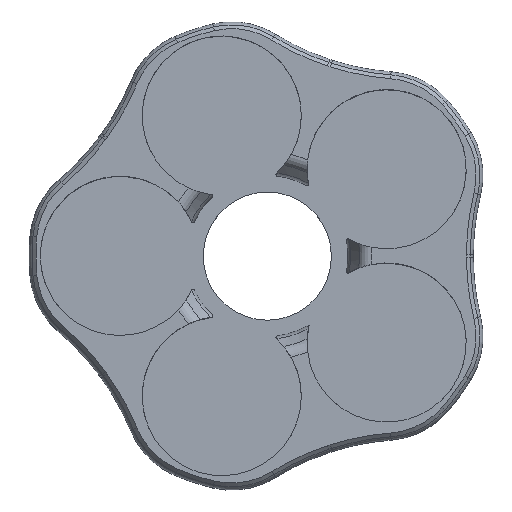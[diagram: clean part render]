
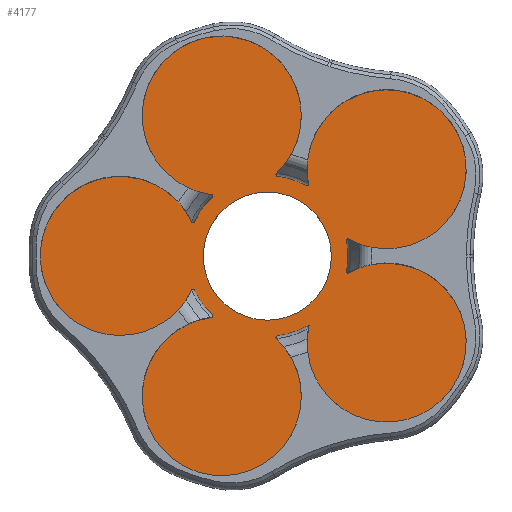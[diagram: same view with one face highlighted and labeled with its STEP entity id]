
A CAD part, top view. The second image highlights one B-rep face of the part: STEP entity #4177.
In plain terms, the highlighted planar face has unit normal (0, 0, 1).
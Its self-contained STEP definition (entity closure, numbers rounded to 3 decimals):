
#107=FACE_BOUND('',#1178,.T.);
#131=PLANE('',#4820);
#906=FACE_OUTER_BOUND('',#1177,.T.);
#1177=EDGE_LOOP('',(#3790,#3791,#3792,#3793,#3794,#3795,#3796,#3797,#3798,
#3799,#3800,#3801,#3802,#3803,#3804,#3805,#3806,#3807,#3808));
#1178=EDGE_LOOP('',(#3809));
#1285=CIRCLE('',#4345,0.1);
#1289=CIRCLE('',#4350,5.775);
#1294=CIRCLE('',#4357,0.1);
#1295=CIRCLE('',#4359,5.775);
#1299=CIRCLE('',#4364,0.1);
#1301=CIRCLE('',#4367,0.1);
#1303=CIRCLE('',#4370,5.85);
#1310=CIRCLE('',#4381,5.775);
#1318=CIRCLE('',#4398,5.775);
#1322=CIRCLE('',#4403,0.1);
#1326=CIRCLE('',#4409,0.1);
#1332=CIRCLE('',#4420,0.1);
#1334=CIRCLE('',#4423,5.85);
#1336=CIRCLE('',#4426,0.1);
#1341=CIRCLE('',#4433,0.1);
#1343=CIRCLE('',#4436,5.775);
#1549=CIRCLE('',#4793,4.65);
#1553=CIRCLE('',#4801,5.85);
#1556=CIRCLE('',#4808,5.85);
#1558=CIRCLE('',#4812,5.85);
#1645=VERTEX_POINT('',#6530);
#1646=VERTEX_POINT('',#6532);
#1662=VERTEX_POINT('',#6606);
#1666=VERTEX_POINT('',#6618);
#1667=VERTEX_POINT('',#6620);
#1668=VERTEX_POINT('',#6624);
#1684=VERTEX_POINT('',#6698);
#1687=VERTEX_POINT('',#6705);
#1688=VERTEX_POINT('',#6707);
#1710=VERTEX_POINT('',#6853);
#1729=VERTEX_POINT('',#7000);
#1730=VERTEX_POINT('',#7002);
#1742=VERTEX_POINT('',#7058);
#1744=VERTEX_POINT('',#7067);
#1756=VERTEX_POINT('',#7138);
#1757=VERTEX_POINT('',#7140);
#1759=VERTEX_POINT('',#7149);
#1763=VERTEX_POINT('',#7161);
#1764=VERTEX_POINT('',#7163);
#1931=VERTEX_POINT('',#8048);
#2060=EDGE_CURVE('',#1645,#1646,#1285,.F.);
#2078=EDGE_CURVE('',#1645,#1662,#1289,.T.);
#2084=EDGE_CURVE('',#1666,#1667,#1294,.F.);
#2086=EDGE_CURVE('',#1668,#1667,#1295,.T.);
#2104=EDGE_CURVE('',#1684,#1662,#1299,.F.);
#2107=EDGE_CURVE('',#1687,#1688,#1301,.F.);
#2110=EDGE_CURVE('',#1688,#1684,#1303,.T.);
#2138=EDGE_CURVE('',#1687,#1710,#1310,.T.);
#2167=EDGE_CURVE('',#1730,#1729,#1318,.T.);
#2181=EDGE_CURVE('',#1742,#1729,#1322,.F.);
#2186=EDGE_CURVE('',#1744,#1710,#1326,.F.);
#2202=EDGE_CURVE('',#1756,#1757,#1332,.F.);
#2205=EDGE_CURVE('',#1757,#1744,#1334,.T.);
#2207=EDGE_CURVE('',#1730,#1759,#1336,.F.);
#2214=EDGE_CURVE('',#1763,#1764,#1341,.F.);
#2225=EDGE_CURVE('',#1756,#1764,#1343,.T.);
#2549=EDGE_CURVE('',#1931,#1931,#1549,.T.);
#2553=EDGE_CURVE('',#1646,#1666,#1553,.T.);
#2556=EDGE_CURVE('',#1668,#1742,#1556,.T.);
#2558=EDGE_CURVE('',#1759,#1763,#1558,.T.);
#3790=ORIENTED_EDGE('',*,*,#2138,.T.);
#3791=ORIENTED_EDGE('',*,*,#2186,.F.);
#3792=ORIENTED_EDGE('',*,*,#2205,.F.);
#3793=ORIENTED_EDGE('',*,*,#2202,.F.);
#3794=ORIENTED_EDGE('',*,*,#2225,.T.);
#3795=ORIENTED_EDGE('',*,*,#2214,.F.);
#3796=ORIENTED_EDGE('',*,*,#2558,.F.);
#3797=ORIENTED_EDGE('',*,*,#2207,.F.);
#3798=ORIENTED_EDGE('',*,*,#2167,.T.);
#3799=ORIENTED_EDGE('',*,*,#2181,.F.);
#3800=ORIENTED_EDGE('',*,*,#2556,.F.);
#3801=ORIENTED_EDGE('',*,*,#2086,.T.);
#3802=ORIENTED_EDGE('',*,*,#2084,.F.);
#3803=ORIENTED_EDGE('',*,*,#2553,.F.);
#3804=ORIENTED_EDGE('',*,*,#2060,.F.);
#3805=ORIENTED_EDGE('',*,*,#2078,.T.);
#3806=ORIENTED_EDGE('',*,*,#2104,.F.);
#3807=ORIENTED_EDGE('',*,*,#2110,.F.);
#3808=ORIENTED_EDGE('',*,*,#2107,.F.);
#3809=ORIENTED_EDGE('',*,*,#2549,.F.);
#4177=ADVANCED_FACE('',(#906,#107),#131,.T.);
#4345=AXIS2_PLACEMENT_3D('',#6533,#5151,#5152);
#4350=AXIS2_PLACEMENT_3D('',#6608,#5167,#5168);
#4357=AXIS2_PLACEMENT_3D('',#6621,#5182,#5183);
#4359=AXIS2_PLACEMENT_3D('',#6625,#5187,#5188);
#4364=AXIS2_PLACEMENT_3D('',#6700,#5203,#5204);
#4367=AXIS2_PLACEMENT_3D('',#6708,#5210,#5211);
#4370=AXIS2_PLACEMENT_3D('',#6712,#5217,#5218);
#4381=AXIS2_PLACEMENT_3D('',#6855,#5246,#5247);
#4398=AXIS2_PLACEMENT_3D('',#7003,#5287,#5288);
#4403=AXIS2_PLACEMENT_3D('',#7060,#5301,#5302);
#4409=AXIS2_PLACEMENT_3D('',#7069,#5314,#5315);
#4420=AXIS2_PLACEMENT_3D('',#7141,#5340,#5341);
#4423=AXIS2_PLACEMENT_3D('',#7145,#5347,#5348);
#4426=AXIS2_PLACEMENT_3D('',#7150,#5353,#5354);
#4433=AXIS2_PLACEMENT_3D('',#7164,#5369,#5370);
#4436=AXIS2_PLACEMENT_3D('',#7216,#5378,#5379);
#4793=AXIS2_PLACEMENT_3D('',#8050,#6198,#6199);
#4801=AXIS2_PLACEMENT_3D('',#8067,#6214,#6215);
#4808=AXIS2_PLACEMENT_3D('',#8083,#6228,#6229);
#4812=AXIS2_PLACEMENT_3D('',#8096,#6236,#6237);
#4820=AXIS2_PLACEMENT_3D('',#8113,#6252,#6253);
#5151=DIRECTION('center_axis',(0.,0.,-1.));
#5152=DIRECTION('ref_axis',(-0.59,0.807,0.));
#5167=DIRECTION('center_axis',(0.,0.,1.));
#5168=DIRECTION('ref_axis',(0.,1.,0.));
#5182=DIRECTION('center_axis',(0.,0.,-1.));
#5183=DIRECTION('ref_axis',(-0.59,-0.807,0.));
#5187=DIRECTION('center_axis',(0.,0.,1.));
#5188=DIRECTION('ref_axis',(0.,1.,0.));
#5203=DIRECTION('center_axis',(0.,0.,-1.));
#5204=DIRECTION('ref_axis',(0.585,-0.811,0.));
#5210=DIRECTION('center_axis',(0.,0.,-1.));
#5211=DIRECTION('ref_axis',(-0.95,-0.312,0.));
#5217=DIRECTION('center_axis',(0.,0.,-1.));
#5218=DIRECTION('ref_axis',(0.,1.,0.));
#5246=DIRECTION('center_axis',(0.,0.,1.));
#5247=DIRECTION('ref_axis',(0.,1.,0.));
#5287=DIRECTION('center_axis',(0.,0.,1.));
#5288=DIRECTION('ref_axis',(0.,1.,0.));
#5301=DIRECTION('center_axis',(0.,0.,-1.));
#5302=DIRECTION('ref_axis',(-0.95,0.312,0.));
#5314=DIRECTION('center_axis',(0.,0.,-1.));
#5315=DIRECTION('ref_axis',(0.952,0.306,0.));
#5340=DIRECTION('center_axis',(0.,0.,-1.));
#5341=DIRECTION('ref_axis',(0.003,-1.,0.));
#5347=DIRECTION('center_axis',(0.,0.,-1.));
#5348=DIRECTION('ref_axis',(0.,1.,0.));
#5353=DIRECTION('center_axis',(0.,0.,-1.));
#5354=DIRECTION('ref_axis',(0.952,-0.306,0.));
#5369=DIRECTION('center_axis',(0.,0.,-1.));
#5370=DIRECTION('ref_axis',(0.003,1.,0.));
#5378=DIRECTION('center_axis',(0.,0.,1.));
#5379=DIRECTION('ref_axis',(0.,1.,0.));
#6198=DIRECTION('center_axis',(0.,0.,1.));
#6199=DIRECTION('ref_axis',(0.,1.,0.));
#6214=DIRECTION('center_axis',(0.,0.,-1.));
#6215=DIRECTION('ref_axis',(0.,1.,0.));
#6228=DIRECTION('center_axis',(0.,0.,-1.));
#6229=DIRECTION('ref_axis',(0.,1.,0.));
#6236=DIRECTION('center_axis',(0.,0.,-1.));
#6237=DIRECTION('ref_axis',(0.,1.,0.));
#6252=DIRECTION('center_axis',(0.,0.,1.));
#6253=DIRECTION('ref_axis',(0.,1.,0.));
#6530=CARTESIAN_POINT('',(-100.411,-9.479,4.));
#6532=CARTESIAN_POINT('',(-100.557,-9.586,4.));
#6533=CARTESIAN_POINT('Origin',(-100.459,-9.567,4.));
#6606=CARTESIAN_POINT('',(-103.319,-5.476,4.));
#6608=CARTESIAN_POINT('Origin',(-97.644,-4.411,4.));
#6618=CARTESIAN_POINT('',(-100.557,-11.814,4.));
#6620=CARTESIAN_POINT('',(-100.411,-11.921,4.));
#6621=CARTESIAN_POINT('Origin',(-100.459,-11.833,4.));
#6624=CARTESIAN_POINT('',(-103.274,-15.707,4.));
#6625=CARTESIAN_POINT('Origin',(-97.644,-16.989,4.));
#6698=CARTESIAN_POINT('',(-103.466,-5.582,4.));
#6700=CARTESIAN_POINT('Origin',(-103.418,-5.495,4.));
#6705=CARTESIAN_POINT('',(-105.641,-4.722,4.));
#6707=CARTESIAN_POINT('',(-105.585,-4.894,4.));
#6708=CARTESIAN_POINT('Origin',(-105.572,-4.795,4.));
#6712=CARTESIAN_POINT('Origin',(-106.3,-10.7,4.));
#6853=CARTESIAN_POINT('',(-110.347,-6.251,4.));
#6855=CARTESIAN_POINT('Origin',(-109.606,-0.524,4.));
#7000=CARTESIAN_POINT('',(-105.641,-16.678,4.));
#7002=CARTESIAN_POINT('',(-110.347,-15.149,4.));
#7003=CARTESIAN_POINT('Origin',(-109.606,-20.876,4.));
#7058=CARTESIAN_POINT('',(-105.585,-16.506,4.));
#7060=CARTESIAN_POINT('Origin',(-105.572,-16.605,4.));
#7067=CARTESIAN_POINT('',(-110.292,-6.423,4.));
#7069=CARTESIAN_POINT('Origin',(-110.36,-6.35,4.));
#7138=CARTESIAN_POINT('',(-111.782,-8.226,4.));
#7140=CARTESIAN_POINT('',(-111.601,-8.225,4.));
#7141=CARTESIAN_POINT('Origin',(-111.691,-8.183,4.));
#7145=CARTESIAN_POINT('Origin',(-106.3,-10.7,4.));
#7149=CARTESIAN_POINT('',(-110.292,-14.977,4.));
#7150=CARTESIAN_POINT('Origin',(-110.36,-15.05,4.));
#7161=CARTESIAN_POINT('',(-111.601,-13.175,4.));
#7163=CARTESIAN_POINT('',(-111.782,-13.174,4.));
#7164=CARTESIAN_POINT('Origin',(-111.691,-13.217,4.));
#7216=CARTESIAN_POINT('Origin',(-117.,-10.7,4.));
#8048=CARTESIAN_POINT('',(-106.3,-15.35,4.));
#8050=CARTESIAN_POINT('Origin',(-106.3,-10.7,4.));
#8067=CARTESIAN_POINT('Origin',(-106.3,-10.7,4.));
#8083=CARTESIAN_POINT('Origin',(-106.3,-10.7,4.));
#8096=CARTESIAN_POINT('Origin',(-106.3,-10.7,4.));
#8113=CARTESIAN_POINT('Origin',(-106.3,-10.7,4.));
